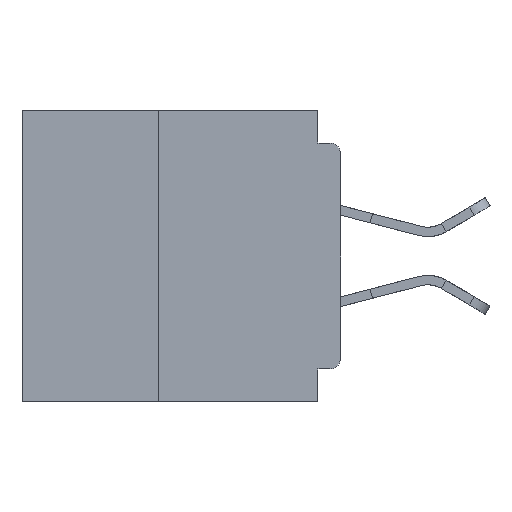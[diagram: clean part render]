
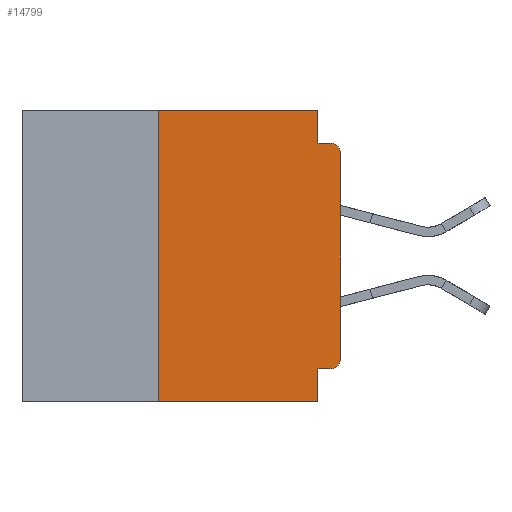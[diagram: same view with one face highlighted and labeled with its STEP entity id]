
A CAD part, left-side view. The second image highlights one B-rep face of the part: STEP entity #14799.
In plain terms, the highlighted planar face has unit normal (-1, 0, 0).
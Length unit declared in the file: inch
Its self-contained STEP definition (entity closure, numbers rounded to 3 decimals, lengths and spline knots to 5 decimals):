
#629 = CARTESIAN_POINT ( 'NONE',  ( 0., 0.031, -0.4 ) ) ;
#806 = CARTESIAN_POINT ( 'NONE',  ( 0., 0.25, -0.4 ) ) ;
#1689 = VECTOR ( 'NONE', #36186, 39.37008 ) ;
#1875 = EDGE_CURVE ( 'NONE', #6181, #26750, #35004, .T. ) ;
#3333 = VERTEX_POINT ( 'NONE', #26043 ) ;
#5377 = ORIENTED_EDGE ( 'NONE', *, *, #16851, .T. ) ;
#6181 = VERTEX_POINT ( 'NONE', #36229 ) ;
#6192 = CARTESIAN_POINT ( 'NONE',  ( 0., 0.015, -0.355 ) ) ;
#6775 = LINE ( 'NONE', #37773, #39085 ) ;
#7108 = LINE ( 'NONE', #37158, #23777 ) ;
#8022 = DIRECTION ( 'NONE',  ( -1., 0., 0. ) ) ;
#9896 = VERTEX_POINT ( 'NONE', #25632 ) ;
#10783 = AXIS2_PLACEMENT_3D ( 'NONE', #10791, #32686, #13990 ) ;
#10791 = CARTESIAN_POINT ( 'NONE',  ( 0., 0.015, -0.34 ) ) ;
#10808 = EDGE_CURVE ( 'NONE', #24457, #6181, #6775, .T. ) ;
#11229 = ORIENTED_EDGE ( 'NONE', *, *, #1875, .F. ) ;
#11325 = EDGE_CURVE ( 'NONE', #3333, #31074, #29761, .T. ) ;
#11347 = CARTESIAN_POINT ( 'NONE',  ( 0., 0.031, -0.045 ) ) ;
#11370 = AXIS2_PLACEMENT_3D ( 'NONE', #26779, #8022, #29904 ) ;
#11394 = CARTESIAN_POINT ( 'NONE',  ( 0., 0.437, 0. ) ) ;
#12317 = DIRECTION ( 'NONE',  ( 0., -1., 0. ) ) ;
#12633 = ORIENTED_EDGE ( 'NONE', *, *, #11325, .T. ) ;
#13313 = CARTESIAN_POINT ( 'NONE',  ( 0., 0.25, -0.4 ) ) ;
#13990 = DIRECTION ( 'NONE',  ( 0., 0., -1. ) ) ;
#14493 = CARTESIAN_POINT ( 'NONE',  ( 0., 0., -0.355 ) ) ;
#14585 = DIRECTION ( 'NONE',  ( 0., 0., -1. ) ) ;
#14799 = ADVANCED_FACE ( 'NONE', ( #17467 ), #26985, .F. ) ;
#15043 = CARTESIAN_POINT ( 'NONE',  ( 0., 0.25, 0. ) ) ;
#15434 = ORIENTED_EDGE ( 'NONE', *, *, #36431, .T. ) ;
#16582 = EDGE_LOOP ( 'NONE', ( #12633, #15434, #39328, #11229, #16715, #18679, #20765, #24250, #27267, #5377 ) ) ;
#16715 = ORIENTED_EDGE ( 'NONE', *, *, #10808, .F. ) ;
#16851 = EDGE_CURVE ( 'NONE', #31476, #3333, #39723, .T. ) ;
#17394 = EDGE_CURVE ( 'NONE', #30140, #24457, #21131, .T. ) ;
#17467 = FACE_OUTER_BOUND ( 'NONE', #16582, .T. ) ;
#18679 = ORIENTED_EDGE ( 'NONE', *, *, #17394, .F. ) ;
#19112 = DIRECTION ( 'NONE',  ( 0., -1., 0. ) ) ;
#20152 = VECTOR ( 'NONE', #35191, 39.37008 ) ;
#20182 = VECTOR ( 'NONE', #12317, 39.37008 ) ;
#20386 = EDGE_CURVE ( 'NONE', #26750, #36904, #36787, .T. ) ;
#20765 = ORIENTED_EDGE ( 'NONE', *, *, #38903, .T. ) ;
#21131 = LINE ( 'NONE', #806, #20152 ) ;
#21195 = VECTOR ( 'NONE', #32066, 39.37008 ) ;
#22336 = VECTOR ( 'NONE', #39303, 39.37008 ) ;
#23303 = LINE ( 'NONE', #14493, #22336 ) ;
#23777 = VECTOR ( 'NONE', #27764, 39.37008 ) ;
#24250 = ORIENTED_EDGE ( 'NONE', *, *, #27741, .F. ) ;
#24457 = VERTEX_POINT ( 'NONE', #15043 ) ;
#24781 = CARTESIAN_POINT ( 'NONE',  ( 0., 0., 0. ) ) ;
#25632 = CARTESIAN_POINT ( 'NONE',  ( 0., 0.031, -0.355 ) ) ;
#26043 = CARTESIAN_POINT ( 'NONE',  ( 0., 0., -0.34 ) ) ;
#26750 = VERTEX_POINT ( 'NONE', #11347 ) ;
#26779 = CARTESIAN_POINT ( 'NONE',  ( 0., 0.015, -0.06 ) ) ;
#26985 = PLANE ( 'NONE',  #39281 ) ;
#27267 = ORIENTED_EDGE ( 'NONE', *, *, #39355, .F. ) ;
#27741 = EDGE_CURVE ( 'NONE', #9896, #32180, #29496, .T. ) ;
#27764 = DIRECTION ( 'NONE',  ( 0., -1., 0. ) ) ;
#27917 = DIRECTION ( 'NONE',  ( 0., 0., 1. ) ) ;
#28491 = CARTESIAN_POINT ( 'NONE',  ( 0., 0.031, -0.4 ) ) ;
#28803 = VECTOR ( 'NONE', #27917, 39.37008 ) ;
#29496 = LINE ( 'NONE', #629, #21195 ) ;
#29761 = LINE ( 'NONE', #24781, #28803 ) ;
#29904 = DIRECTION ( 'NONE',  ( 0., 0., -1. ) ) ;
#30140 = VERTEX_POINT ( 'NONE', #13313 ) ;
#30493 = CARTESIAN_POINT ( 'NONE',  ( 0., 0.015, -0.045 ) ) ;
#30841 = CIRCLE ( 'NONE', #11370, 0.015 ) ;
#31074 = VERTEX_POINT ( 'NONE', #38928 ) ;
#31476 = VERTEX_POINT ( 'NONE', #6192 ) ;
#32066 = DIRECTION ( 'NONE',  ( 0., 0., -1. ) ) ;
#32180 = VERTEX_POINT ( 'NONE', #28491 ) ;
#32686 = DIRECTION ( 'NONE',  ( -1., 0., 0. ) ) ;
#33276 = DIRECTION ( 'NONE',  ( 1., 0., 0. ) ) ;
#35004 = LINE ( 'NONE', #36372, #1689 ) ;
#35191 = DIRECTION ( 'NONE',  ( 0., 0., 1. ) ) ;
#36186 = DIRECTION ( 'NONE',  ( 0., 0., -1. ) ) ;
#36229 = CARTESIAN_POINT ( 'NONE',  ( 0., 0.031, 0. ) ) ;
#36372 = CARTESIAN_POINT ( 'NONE',  ( 0., 0.031, 0. ) ) ;
#36431 = EDGE_CURVE ( 'NONE', #31074, #36904, #30841, .T. ) ;
#36787 = LINE ( 'NONE', #37316, #20182 ) ;
#36904 = VERTEX_POINT ( 'NONE', #30493 ) ;
#37158 = CARTESIAN_POINT ( 'NONE',  ( 0., 0.437, -0.4 ) ) ;
#37316 = CARTESIAN_POINT ( 'NONE',  ( 0., 0., -0.045 ) ) ;
#37773 = CARTESIAN_POINT ( 'NONE',  ( 0., 0.437, 0. ) ) ;
#38903 = EDGE_CURVE ( 'NONE', #30140, #32180, #7108, .T. ) ;
#38928 = CARTESIAN_POINT ( 'NONE',  ( 0., 0., -0.06 ) ) ;
#39085 = VECTOR ( 'NONE', #19112, 39.37008 ) ;
#39281 = AXIS2_PLACEMENT_3D ( 'NONE', #11394, #33276, #14585 ) ;
#39303 = DIRECTION ( 'NONE',  ( 0., 1., 0. ) ) ;
#39328 = ORIENTED_EDGE ( 'NONE', *, *, #20386, .F. ) ;
#39355 = EDGE_CURVE ( 'NONE', #31476, #9896, #23303, .T. ) ;
#39723 = CIRCLE ( 'NONE', #10783, 0.015 ) ;
